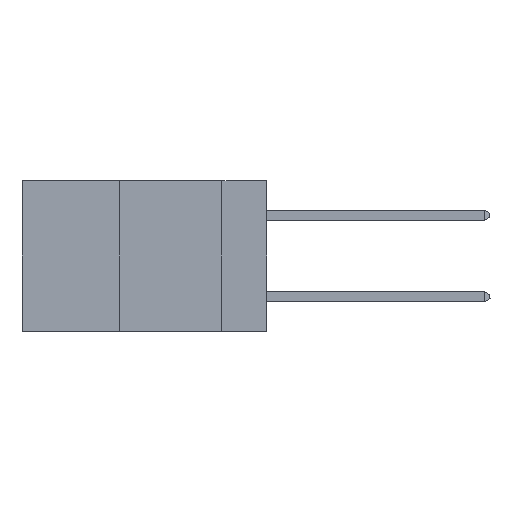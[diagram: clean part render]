
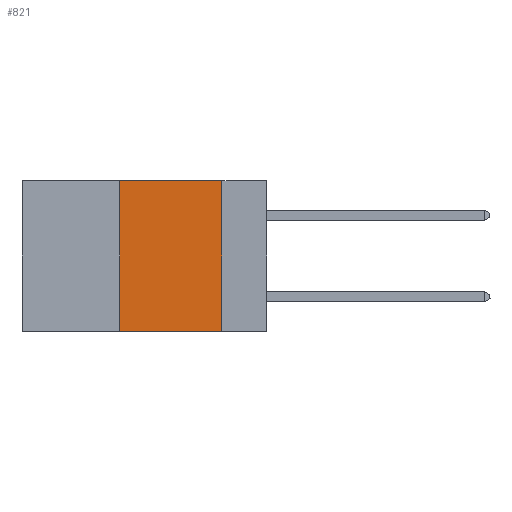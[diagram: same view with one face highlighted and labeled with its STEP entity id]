
A CAD part, left-side view. The second image highlights one B-rep face of the part: STEP entity #821.
In plain terms, the highlighted planar face has unit normal (-1, 0, 0).
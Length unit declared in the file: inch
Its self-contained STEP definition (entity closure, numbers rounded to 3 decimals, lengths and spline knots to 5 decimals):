
#198 = CARTESIAN_POINT ( 'NONE',  ( 0., 0.6, -0.37 ) ) ;
#821 = ADVANCED_FACE ( 'NONE', ( #25411 ), #27713, .F. ) ;
#878 = CARTESIAN_POINT ( 'NONE',  ( 0., 0.36, 0. ) ) ;
#1095 = DIRECTION ( 'NONE',  ( 0., 0., -1. ) ) ;
#2264 = DIRECTION ( 'NONE',  ( 1., 0., 0. ) ) ;
#2937 = ORIENTED_EDGE ( 'NONE', *, *, #5345, .F. ) ;
#3008 = CARTESIAN_POINT ( 'NONE',  ( 0., 0.6, 0. ) ) ;
#3303 = LINE ( 'NONE', #3008, #14071 ) ;
#3308 = AXIS2_PLACEMENT_3D ( 'NONE', #19166, #2264, #4321 ) ;
#4321 = DIRECTION ( 'NONE',  ( 0., 0., -1. ) ) ;
#5345 = EDGE_CURVE ( 'NONE', #10378, #18418, #3303, .T. ) ;
#7390 = VECTOR ( 'NONE', #20321, 39.37008 ) ;
#8256 = EDGE_CURVE ( 'NONE', #11025, #12129, #26107, .T. ) ;
#10378 = VERTEX_POINT ( 'NONE', #13978 ) ;
#10980 = EDGE_CURVE ( 'NONE', #11025, #10378, #13119, .T. ) ;
#11025 = VERTEX_POINT ( 'NONE', #11784 ) ;
#11528 = CARTESIAN_POINT ( 'NONE',  ( 0., 0.11, 0. ) ) ;
#11784 = CARTESIAN_POINT ( 'NONE',  ( 0., 0.36, -0.37 ) ) ;
#12129 = VERTEX_POINT ( 'NONE', #26237 ) ;
#13119 = LINE ( 'NONE', #878, #7390 ) ;
#13558 = VECTOR ( 'NONE', #1095, 39.37008 ) ;
#13978 = CARTESIAN_POINT ( 'NONE',  ( 0., 0.36, 0. ) ) ;
#14071 = VECTOR ( 'NONE', #18040, 39.37008 ) ;
#15072 = ORIENTED_EDGE ( 'NONE', *, *, #10980, .F. ) ;
#16166 = EDGE_CURVE ( 'NONE', #18418, #12129, #22632, .T. ) ;
#17761 = ORIENTED_EDGE ( 'NONE', *, *, #16166, .F. ) ;
#18040 = DIRECTION ( 'NONE',  ( 0., -1., 0. ) ) ;
#18418 = VERTEX_POINT ( 'NONE', #24158 ) ;
#19166 = CARTESIAN_POINT ( 'NONE',  ( 0., 0.6, 0. ) ) ;
#19473 = DIRECTION ( 'NONE',  ( 0., -1., 0. ) ) ;
#20073 = ORIENTED_EDGE ( 'NONE', *, *, #8256, .T. ) ;
#20321 = DIRECTION ( 'NONE',  ( 0., 0., 1. ) ) ;
#22632 = LINE ( 'NONE', #11528, #13558 ) ;
#23411 = EDGE_LOOP ( 'NONE', ( #17761, #2937, #15072, #20073 ) ) ;
#24158 = CARTESIAN_POINT ( 'NONE',  ( 0., 0.11, 0. ) ) ;
#25411 = FACE_OUTER_BOUND ( 'NONE', #23411, .T. ) ;
#26107 = LINE ( 'NONE', #198, #27124 ) ;
#26237 = CARTESIAN_POINT ( 'NONE',  ( 0., 0.11, -0.37 ) ) ;
#27124 = VECTOR ( 'NONE', #19473, 39.37008 ) ;
#27713 = PLANE ( 'NONE',  #3308 ) ;
